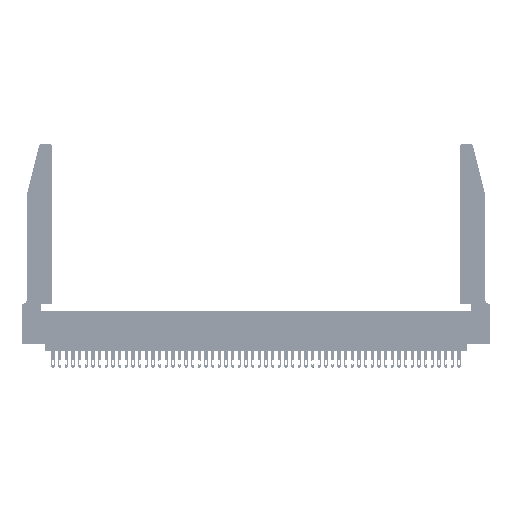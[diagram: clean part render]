
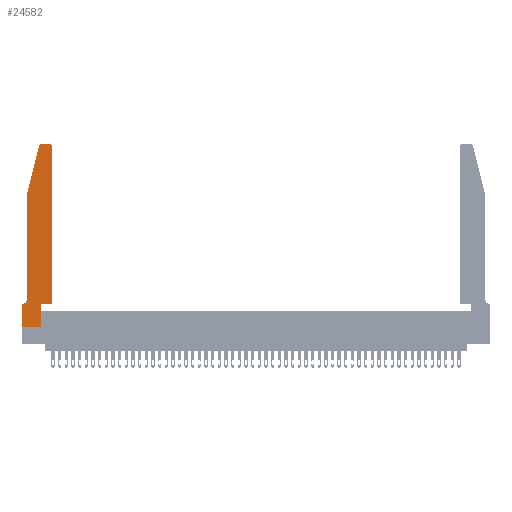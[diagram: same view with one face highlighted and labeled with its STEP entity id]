
A CAD part, top view. The second image highlights one B-rep face of the part: STEP entity #24582.
In plain terms, the highlighted planar face has unit normal (0, 0, 1).
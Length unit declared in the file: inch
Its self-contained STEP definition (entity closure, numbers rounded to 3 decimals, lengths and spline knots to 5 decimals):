
#271 = CARTESIAN_POINT ( 'NONE',  ( 0.2865, 0.35, 0.37 ) ) ;
#611 = LINE ( 'NONE', #271, #29483 ) ;
#880 = EDGE_CURVE ( 'NONE', #17751, #30698, #20720, .T. ) ;
#1096 = EDGE_CURVE ( 'NONE', #35855, #2512, #23178, .T. ) ;
#1144 = CARTESIAN_POINT ( 'NONE',  ( 0., 0., 0.37 ) ) ;
#1528 = LINE ( 'NONE', #10496, #29772 ) ;
#2094 = VERTEX_POINT ( 'NONE', #38849 ) ;
#2347 = VECTOR ( 'NONE', #23124, 39.37008 ) ;
#2351 = CIRCLE ( 'NONE', #25786, 0.07 ) ;
#2512 = VERTEX_POINT ( 'NONE', #1144 ) ;
#2796 = VERTEX_POINT ( 'NONE', #21072 ) ;
#3892 = DIRECTION ( 'NONE',  ( -1., 0., 0. ) ) ;
#4296 = EDGE_CURVE ( 'NONE', #50250, #25120, #8564, .T. ) ;
#5535 = CARTESIAN_POINT ( 'NONE',  ( 0., 0.35, 0.37 ) ) ;
#5975 = DIRECTION ( 'NONE',  ( 0., 0., 1. ) ) ;
#6346 = CARTESIAN_POINT ( 'NONE',  ( 0.284, 2.75, 0.37 ) ) ;
#7063 = AXIS2_PLACEMENT_3D ( 'NONE', #5535, #36227, #44316 ) ;
#7836 = ORIENTED_EDGE ( 'NONE', *, *, #23704, .T. ) ;
#8564 = CIRCLE ( 'NONE', #21384, 0.03 ) ;
#10092 = CIRCLE ( 'NONE', #45019, 0.03 ) ;
#10306 = VECTOR ( 'NONE', #22826, 39.37008 ) ;
#10496 = CARTESIAN_POINT ( 'NONE',  ( 0.0755, 2., 0.37 ) ) ;
#10517 = EDGE_CURVE ( 'NONE', #33678, #17751, #611, .T. ) ;
#11092 = CARTESIAN_POINT ( 'NONE',  ( 0.0055, 0.35, 0.37 ) ) ;
#11566 = ORIENTED_EDGE ( 'NONE', *, *, #20935, .T. ) ;
#12079 = CARTESIAN_POINT ( 'NONE',  ( 0.0755, 0.35, 0.37 ) ) ;
#13904 = EDGE_CURVE ( 'NONE', #30698, #2094, #26678, .T. ) ;
#14410 = VECTOR ( 'NONE', #46793, 39.37008 ) ;
#15010 = CARTESIAN_POINT ( 'NONE',  ( 0.0055, 0.42, 0.37 ) ) ;
#15347 = DIRECTION ( 'NONE',  ( 0., 0., -1. ) ) ;
#16298 = ORIENTED_EDGE ( 'NONE', *, *, #34096, .T. ) ;
#17393 = CARTESIAN_POINT ( 'NONE',  ( 0.0755, 2., 0.37 ) ) ;
#17751 = VERTEX_POINT ( 'NONE', #29661 ) ;
#17938 = CARTESIAN_POINT ( 'NONE',  ( 0.2605, 2.75, 0.37 ) ) ;
#18729 = ORIENTED_EDGE ( 'NONE', *, *, #19947, .T. ) ;
#19678 = ORIENTED_EDGE ( 'NONE', *, *, #880, .T. ) ;
#19930 = CARTESIAN_POINT ( 'NONE',  ( 0.4505, 0.35, 0.37 ) ) ;
#19947 = EDGE_CURVE ( 'NONE', #2512, #33678, #21771, .T. ) ;
#20720 = LINE ( 'NONE', #23488, #10306 ) ;
#20935 = EDGE_CURVE ( 'NONE', #2796, #33336, #1528, .T. ) ;
#21072 = CARTESIAN_POINT ( 'NONE',  ( 0.0755, 2., 0.37 ) ) ;
#21384 = AXIS2_PLACEMENT_3D ( 'NONE', #23456, #27113, #31028 ) ;
#21771 = LINE ( 'NONE', #38539, #14410 ) ;
#21790 = VERTEX_POINT ( 'NONE', #47293 ) ;
#21797 = EDGE_LOOP ( 'NONE', ( #16298, #30602, #41468, #11566, #7836, #45711, #42249, #18729, #45423, #19678, #31382, #48941 ) ) ;
#22826 = DIRECTION ( 'NONE',  ( 1., 0., 0. ) ) ;
#23124 = DIRECTION ( 'NONE',  ( 0., -1., 0. ) ) ;
#23178 = LINE ( 'NONE', #38745, #2347 ) ;
#23456 = CARTESIAN_POINT ( 'NONE',  ( 0.284, 2.72, 0.37 ) ) ;
#23488 = CARTESIAN_POINT ( 'NONE',  ( 0.4505, 0.35, 0.37 ) ) ;
#23522 = VECTOR ( 'NONE', #48416, 39.37008 ) ;
#23677 = VERTEX_POINT ( 'NONE', #11092 ) ;
#23704 = EDGE_CURVE ( 'NONE', #33336, #23677, #2351, .T. ) ;
#24582 = ADVANCED_FACE ( 'NONE', ( #35328 ), #40184, .T. ) ;
#25120 = VERTEX_POINT ( 'NONE', #43381 ) ;
#25786 = AXIS2_PLACEMENT_3D ( 'NONE', #15010, #15347, #42825 ) ;
#26266 = VECTOR ( 'NONE', #45782, 39.37008 ) ;
#26678 = LINE ( 'NONE', #19930, #23522 ) ;
#27113 = DIRECTION ( 'NONE',  ( 0., 0., 1. ) ) ;
#29483 = VECTOR ( 'NONE', #44386, 39.37008 ) ;
#29621 = DIRECTION ( 'NONE',  ( 1., 0., 0. ) ) ;
#29661 = CARTESIAN_POINT ( 'NONE',  ( 0.2865, 0.35, 0.37 ) ) ;
#29711 = DIRECTION ( 'NONE',  ( 0., -1., 0. ) ) ;
#29724 = EDGE_CURVE ( 'NONE', #2094, #21790, #10092, .T. ) ;
#29772 = VECTOR ( 'NONE', #29711, 39.37008 ) ;
#30602 = ORIENTED_EDGE ( 'NONE', *, *, #4296, .T. ) ;
#30698 = VERTEX_POINT ( 'NONE', #43960 ) ;
#31028 = DIRECTION ( 'NONE',  ( 1., 0., 0. ) ) ;
#31382 = ORIENTED_EDGE ( 'NONE', *, *, #13904, .T. ) ;
#33336 = VERTEX_POINT ( 'NONE', #36238 ) ;
#33678 = VERTEX_POINT ( 'NONE', #46011 ) ;
#34096 = EDGE_CURVE ( 'NONE', #21790, #50250, #38538, .T. ) ;
#35328 = FACE_OUTER_BOUND ( 'NONE', #21797, .T. ) ;
#35855 = VERTEX_POINT ( 'NONE', #41069 ) ;
#36227 = DIRECTION ( 'NONE',  ( 0., 0., 1. ) ) ;
#36238 = CARTESIAN_POINT ( 'NONE',  ( 0.0755, 0.42, 0.37 ) ) ;
#37154 = CARTESIAN_POINT ( 'NONE',  ( 0.4205, 2.72, 0.37 ) ) ;
#38014 = VECTOR ( 'NONE', #48649, 39.37008 ) ;
#38538 = LINE ( 'NONE', #17938, #26266 ) ;
#38539 = CARTESIAN_POINT ( 'NONE',  ( 0., 0., 0.37 ) ) ;
#38693 = EDGE_CURVE ( 'NONE', #23677, #35855, #42526, .T. ) ;
#38745 = CARTESIAN_POINT ( 'NONE',  ( 0., 0., 0.37 ) ) ;
#38849 = CARTESIAN_POINT ( 'NONE',  ( 0.4505, 2.72, 0.37 ) ) ;
#40184 = PLANE ( 'NONE',  #7063 ) ;
#41069 = CARTESIAN_POINT ( 'NONE',  ( 0., 0.35, 0.37 ) ) ;
#41309 = VECTOR ( 'NONE', #3892, 39.37008 ) ;
#41468 = ORIENTED_EDGE ( 'NONE', *, *, #43793, .T. ) ;
#42249 = ORIENTED_EDGE ( 'NONE', *, *, #1096, .T. ) ;
#42526 = LINE ( 'NONE', #12079, #41309 ) ;
#42825 = DIRECTION ( 'NONE',  ( -1., 0., 0. ) ) ;
#43381 = CARTESIAN_POINT ( 'NONE',  ( 0.25487, 2.72718, 0.37 ) ) ;
#43793 = EDGE_CURVE ( 'NONE', #25120, #2796, #49674, .T. ) ;
#43960 = CARTESIAN_POINT ( 'NONE',  ( 0.4505, 0.35, 0.37 ) ) ;
#44316 = DIRECTION ( 'NONE',  ( 1., 0., 0. ) ) ;
#44386 = DIRECTION ( 'NONE',  ( 0., 1., 0. ) ) ;
#45019 = AXIS2_PLACEMENT_3D ( 'NONE', #37154, #5975, #29621 ) ;
#45423 = ORIENTED_EDGE ( 'NONE', *, *, #10517, .T. ) ;
#45711 = ORIENTED_EDGE ( 'NONE', *, *, #38693, .T. ) ;
#45782 = DIRECTION ( 'NONE',  ( -1., 0., 0. ) ) ;
#46011 = CARTESIAN_POINT ( 'NONE',  ( 0.2865, 0., 0.37 ) ) ;
#46793 = DIRECTION ( 'NONE',  ( 1., 0., 0. ) ) ;
#47293 = CARTESIAN_POINT ( 'NONE',  ( 0.4205, 2.75, 0.37 ) ) ;
#48416 = DIRECTION ( 'NONE',  ( 0., 1., 0. ) ) ;
#48649 = DIRECTION ( 'NONE',  ( -0.239, -0.971, 0. ) ) ;
#48941 = ORIENTED_EDGE ( 'NONE', *, *, #29724, .T. ) ;
#49674 = LINE ( 'NONE', #17393, #38014 ) ;
#50250 = VERTEX_POINT ( 'NONE', #6346 ) ;
